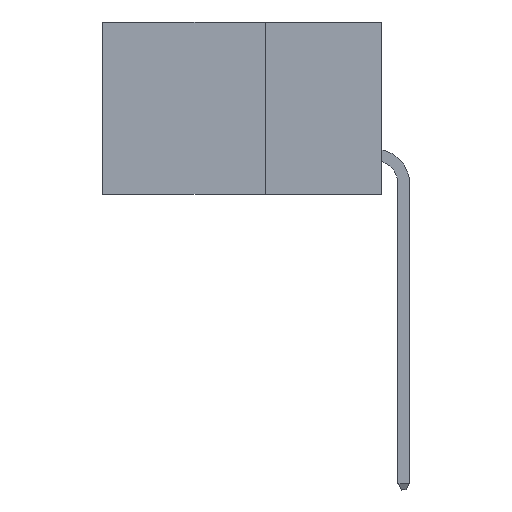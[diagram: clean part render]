
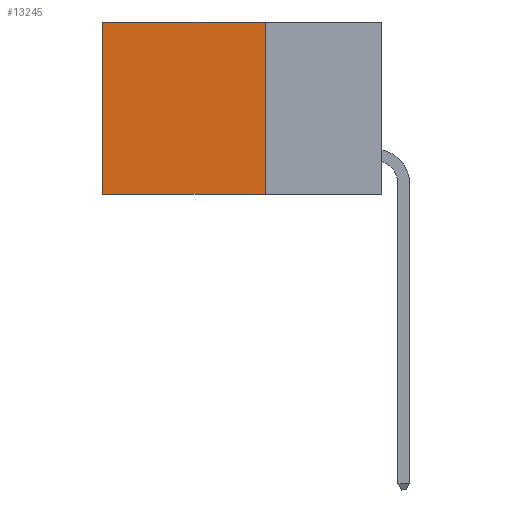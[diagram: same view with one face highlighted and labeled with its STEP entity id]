
A CAD part, left-side view. The second image highlights one B-rep face of the part: STEP entity #13245.
In plain terms, the highlighted planar face has unit normal (-1, 0, 0).
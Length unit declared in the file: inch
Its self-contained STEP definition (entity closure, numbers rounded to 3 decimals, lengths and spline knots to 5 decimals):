
#656 = VECTOR ( 'NONE', #11675, 39.37008 ) ;
#1263 = ORIENTED_EDGE ( 'NONE', *, *, #8286, .F. ) ;
#2892 = DIRECTION ( 'NONE',  ( 0., 1., 0. ) ) ;
#3257 = VECTOR ( 'NONE', #2892, 39.37008 ) ;
#3410 = CARTESIAN_POINT ( 'NONE',  ( 0.2875, 0.25, 0. ) ) ;
#4598 = EDGE_CURVE ( 'NONE', #12176, #19332, #10091, .T. ) ;
#6114 = CARTESIAN_POINT ( 'NONE',  ( 0.2875, 0.6, 0. ) ) ;
#6638 = VECTOR ( 'NONE', #22671, 39.37008 ) ;
#7125 = EDGE_CURVE ( 'NONE', #11489, #19332, #9996, .T. ) ;
#7295 = VERTEX_POINT ( 'NONE', #11847 ) ;
#7465 = ORIENTED_EDGE ( 'NONE', *, *, #12810, .T. ) ;
#8286 = EDGE_CURVE ( 'NONE', #7295, #12176, #15288, .T. ) ;
#8437 = FACE_OUTER_BOUND ( 'NONE', #12630, .T. ) ;
#9996 = LINE ( 'NONE', #11660, #20255 ) ;
#10091 = LINE ( 'NONE', #17458, #6638 ) ;
#11489 = VERTEX_POINT ( 'NONE', #6114 ) ;
#11660 = CARTESIAN_POINT ( 'NONE',  ( 0.2875, 0.6, 0. ) ) ;
#11675 = DIRECTION ( 'NONE',  ( 0., 0., -1. ) ) ;
#11847 = CARTESIAN_POINT ( 'NONE',  ( 0.2875, 0.25, 0. ) ) ;
#12176 = VERTEX_POINT ( 'NONE', #14776 ) ;
#12630 = EDGE_LOOP ( 'NONE', ( #20609, #21542, #1263, #7465 ) ) ;
#12810 = EDGE_CURVE ( 'NONE', #7295, #11489, #19627, .T. ) ;
#13245 = ADVANCED_FACE ( 'NONE', ( #8437 ), #14393, .F. ) ;
#14393 = PLANE ( 'NONE',  #17991 ) ;
#14776 = CARTESIAN_POINT ( 'NONE',  ( 0.2875, 0.25, -0.37 ) ) ;
#15288 = LINE ( 'NONE', #19129, #656 ) ;
#16215 = DIRECTION ( 'NONE',  ( 1., 0., 0. ) ) ;
#16302 = DIRECTION ( 'NONE',  ( 0., 0., -1. ) ) ;
#17019 = DIRECTION ( 'NONE',  ( 0., 0., -1. ) ) ;
#17458 = CARTESIAN_POINT ( 'NONE',  ( 0.2875, 0.25, -0.37 ) ) ;
#17991 = AXIS2_PLACEMENT_3D ( 'NONE', #3410, #16215, #16302 ) ;
#18714 = CARTESIAN_POINT ( 'NONE',  ( 0.2875, 0.25, 0. ) ) ;
#18906 = CARTESIAN_POINT ( 'NONE',  ( 0.2875, 0.6, -0.37 ) ) ;
#19129 = CARTESIAN_POINT ( 'NONE',  ( 0.2875, 0.25, 0. ) ) ;
#19332 = VERTEX_POINT ( 'NONE', #18906 ) ;
#19627 = LINE ( 'NONE', #18714, #3257 ) ;
#20255 = VECTOR ( 'NONE', #17019, 39.37008 ) ;
#20609 = ORIENTED_EDGE ( 'NONE', *, *, #7125, .T. ) ;
#21542 = ORIENTED_EDGE ( 'NONE', *, *, #4598, .F. ) ;
#22671 = DIRECTION ( 'NONE',  ( 0., 1., 0. ) ) ;
